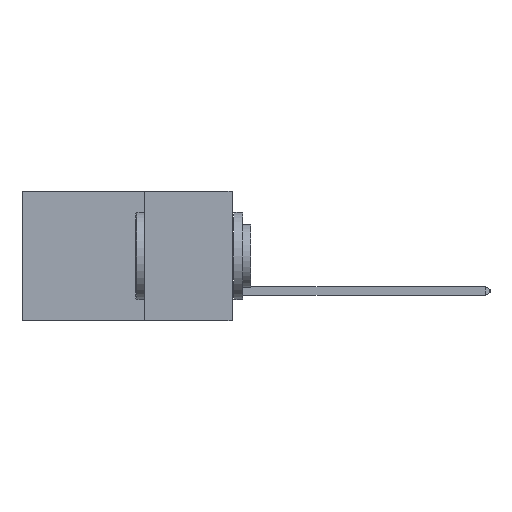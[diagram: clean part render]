
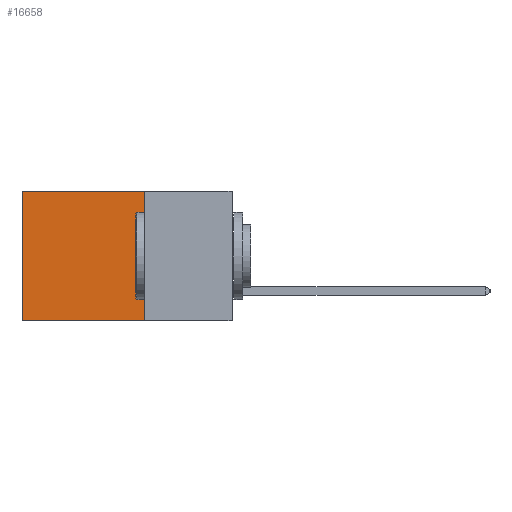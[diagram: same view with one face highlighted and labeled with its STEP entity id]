
A CAD part, left-side view. The second image highlights one B-rep face of the part: STEP entity #16658.
In plain terms, the highlighted planar face has unit normal (-1, 0, 0).
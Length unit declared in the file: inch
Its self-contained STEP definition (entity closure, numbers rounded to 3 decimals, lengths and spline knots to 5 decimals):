
#309 = LINE ( 'NONE', #5736, #20845 ) ;
#1006 = FACE_OUTER_BOUND ( 'NONE', #6419, .T. ) ;
#1496 = CARTESIAN_POINT ( 'NONE',  ( 0.2875, 0.25, 0. ) ) ;
#4280 = LINE ( 'NONE', #16204, #8019 ) ;
#4405 = ORIENTED_EDGE ( 'NONE', *, *, #13502, .T. ) ;
#4808 = DIRECTION ( 'NONE',  ( 1., 0., 0. ) ) ;
#5270 = CARTESIAN_POINT ( 'NONE',  ( 0.2875, 0.25, 0. ) ) ;
#5566 = VERTEX_POINT ( 'NONE', #6703 ) ;
#5736 = CARTESIAN_POINT ( 'NONE',  ( 0.2875, 0.6, 0. ) ) ;
#6221 = VECTOR ( 'NONE', #15877, 39.37008 ) ;
#6315 = EDGE_CURVE ( 'NONE', #20259, #22335, #15892, .T. ) ;
#6419 = EDGE_LOOP ( 'NONE', ( #4405, #21067, #15647, #9024 ) ) ;
#6703 = CARTESIAN_POINT ( 'NONE',  ( 0.2875, 0.25, -0.37 ) ) ;
#6833 = CARTESIAN_POINT ( 'NONE',  ( 0.2875, 0.25, 0. ) ) ;
#7851 = LINE ( 'NONE', #5270, #21253 ) ;
#8019 = VECTOR ( 'NONE', #9002, 39.37008 ) ;
#9002 = DIRECTION ( 'NONE',  ( 0., 1., 0. ) ) ;
#9024 = ORIENTED_EDGE ( 'NONE', *, *, #6315, .T. ) ;
#10325 = EDGE_CURVE ( 'NONE', #5566, #12371, #4280, .T. ) ;
#10459 = AXIS2_PLACEMENT_3D ( 'NONE', #21171, #4808, #17547 ) ;
#12371 = VERTEX_POINT ( 'NONE', #18601 ) ;
#13155 = CARTESIAN_POINT ( 'NONE',  ( 0.2875, 0.6, 0. ) ) ;
#13502 = EDGE_CURVE ( 'NONE', #22335, #12371, #309, .T. ) ;
#14363 = DIRECTION ( 'NONE',  ( 0., 0., -1. ) ) ;
#15647 = ORIENTED_EDGE ( 'NONE', *, *, #16812, .F. ) ;
#15877 = DIRECTION ( 'NONE',  ( 0., 1., 0. ) ) ;
#15892 = LINE ( 'NONE', #6833, #6221 ) ;
#16204 = CARTESIAN_POINT ( 'NONE',  ( 0.2875, 0.25, -0.37 ) ) ;
#16658 = ADVANCED_FACE ( 'NONE', ( #1006 ), #23003, .F. ) ;
#16812 = EDGE_CURVE ( 'NONE', #20259, #5566, #7851, .T. ) ;
#17547 = DIRECTION ( 'NONE',  ( 0., 0., -1. ) ) ;
#18479 = DIRECTION ( 'NONE',  ( 0., 0., -1. ) ) ;
#18601 = CARTESIAN_POINT ( 'NONE',  ( 0.2875, 0.6, -0.37 ) ) ;
#20259 = VERTEX_POINT ( 'NONE', #1496 ) ;
#20845 = VECTOR ( 'NONE', #18479, 39.37008 ) ;
#21067 = ORIENTED_EDGE ( 'NONE', *, *, #10325, .F. ) ;
#21171 = CARTESIAN_POINT ( 'NONE',  ( 0.2875, 0.25, 0. ) ) ;
#21253 = VECTOR ( 'NONE', #14363, 39.37008 ) ;
#22335 = VERTEX_POINT ( 'NONE', #13155 ) ;
#23003 = PLANE ( 'NONE',  #10459 ) ;
